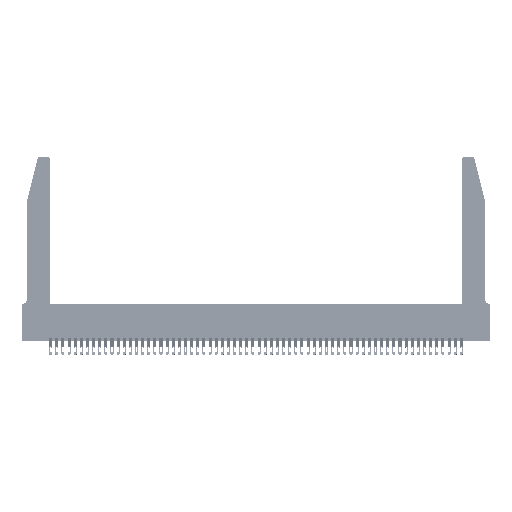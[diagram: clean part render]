
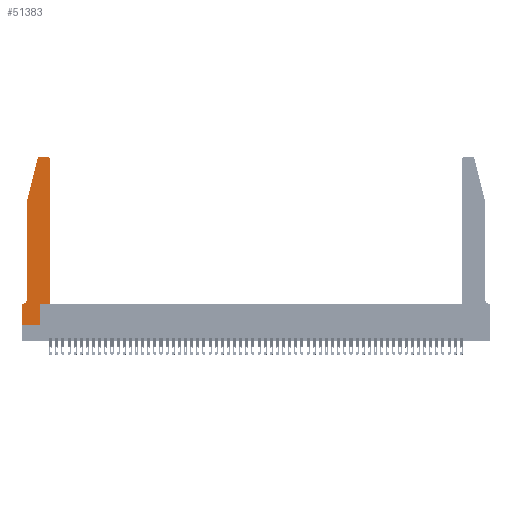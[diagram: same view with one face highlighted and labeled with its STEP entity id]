
A CAD part, top view. The second image highlights one B-rep face of the part: STEP entity #51383.
In plain terms, the highlighted planar face has unit normal (0, 0, 1).
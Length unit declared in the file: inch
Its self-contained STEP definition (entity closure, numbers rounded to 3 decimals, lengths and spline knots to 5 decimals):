
#634 = DIRECTION ( 'NONE',  ( 1., 0., 0. ) ) ;
#1074 = DIRECTION ( 'NONE',  ( -1., 0., 0. ) ) ;
#1122 = EDGE_CURVE ( 'NONE', #22611, #48524, #22011, .T. ) ;
#1380 = LINE ( 'NONE', #47984, #33876 ) ;
#1394 = DIRECTION ( 'NONE',  ( 1., 0., 0. ) ) ;
#1441 = DIRECTION ( 'NONE',  ( 1., 0., 0. ) ) ;
#1552 = EDGE_CURVE ( 'NONE', #48524, #32645, #35868, .T. ) ;
#1897 = DIRECTION ( 'NONE',  ( 1., 0., 0. ) ) ;
#2033 = LINE ( 'NONE', #38883, #20608 ) ;
#2248 = ORIENTED_EDGE ( 'NONE', *, *, #34589, .T. ) ;
#4146 = CARTESIAN_POINT ( 'NONE',  ( 0.4205, 2.75, 0.37 ) ) ;
#4470 = DIRECTION ( 'NONE',  ( 0., -1., 0. ) ) ;
#5925 = CARTESIAN_POINT ( 'NONE',  ( 0.4505, 0.35, 0.37 ) ) ;
#6037 = CARTESIAN_POINT ( 'NONE',  ( 0.0755, 2., 0.37 ) ) ;
#6945 = CARTESIAN_POINT ( 'NONE',  ( 0., 0., 0.37 ) ) ;
#9640 = VECTOR ( 'NONE', #28130, 39.37008 ) ;
#9688 = CARTESIAN_POINT ( 'NONE',  ( 0.4505, 2.72, 0.37 ) ) ;
#9996 = DIRECTION ( 'NONE',  ( 0., 0., 1. ) ) ;
#10215 = CARTESIAN_POINT ( 'NONE',  ( 0.2865, 0.35, 0.37 ) ) ;
#10845 = VERTEX_POINT ( 'NONE', #4146 ) ;
#10889 = LINE ( 'NONE', #16915, #42019 ) ;
#11600 = EDGE_CURVE ( 'NONE', #10845, #16654, #2033, .T. ) ;
#11763 = VECTOR ( 'NONE', #35792, 39.37008 ) ;
#12151 = CARTESIAN_POINT ( 'NONE',  ( 0., 0.35, 0.37 ) ) ;
#13722 = AXIS2_PLACEMENT_3D ( 'NONE', #47189, #35130, #1394 ) ;
#14450 = DIRECTION ( 'NONE',  ( 0., 1., 0. ) ) ;
#14862 = VECTOR ( 'NONE', #52957, 39.37008 ) ;
#14934 = LINE ( 'NONE', #52282, #9640 ) ;
#15047 = DIRECTION ( 'NONE',  ( 0., 0., 1. ) ) ;
#15683 = DIRECTION ( 'NONE',  ( 0., 0., -1. ) ) ;
#15743 = LINE ( 'NONE', #48577, #11763 ) ;
#16171 = CIRCLE ( 'NONE', #44896, 0.03 ) ;
#16654 = VERTEX_POINT ( 'NONE', #47803 ) ;
#16915 = CARTESIAN_POINT ( 'NONE',  ( 0.0755, 0.35, 0.37 ) ) ;
#19220 = FACE_OUTER_BOUND ( 'NONE', #26152, .T. ) ;
#20519 = VERTEX_POINT ( 'NONE', #49483 ) ;
#20608 = VECTOR ( 'NONE', #1074, 39.37008 ) ;
#20613 = CARTESIAN_POINT ( 'NONE',  ( 0.4505, 0.35, 0.37 ) ) ;
#21915 = LINE ( 'NONE', #5925, #41755 ) ;
#22011 = LINE ( 'NONE', #51734, #51879 ) ;
#22611 = VERTEX_POINT ( 'NONE', #27325 ) ;
#22914 = EDGE_CURVE ( 'NONE', #40343, #46086, #21915, .T. ) ;
#25844 = ORIENTED_EDGE ( 'NONE', *, *, #22914, .T. ) ;
#25861 = CARTESIAN_POINT ( 'NONE',  ( 0.4505, 0.35, 0.37 ) ) ;
#26067 = PLANE ( 'NONE',  #13722 ) ;
#26152 = EDGE_LOOP ( 'NONE', ( #49220, #48592, #42575, #53162, #42319, #46544, #34204, #2248, #26347, #48684, #25844, #44415 ) ) ;
#26347 = ORIENTED_EDGE ( 'NONE', *, *, #44273, .T. ) ;
#26510 = VERTEX_POINT ( 'NONE', #45526 ) ;
#26531 = VERTEX_POINT ( 'NONE', #12151 ) ;
#27325 = CARTESIAN_POINT ( 'NONE',  ( 0.0755, 2., 0.37 ) ) ;
#28130 = DIRECTION ( 'NONE',  ( 1., 0., 0. ) ) ;
#30059 = DIRECTION ( 'NONE',  ( -1., 0., 0. ) ) ;
#31421 = EDGE_CURVE ( 'NONE', #53577, #40343, #33157, .T. ) ;
#31683 = DIRECTION ( 'NONE',  ( 0., -1., 0. ) ) ;
#31684 = CIRCLE ( 'NONE', #46049, 0.03 ) ;
#32095 = LINE ( 'NONE', #6037, #14862 ) ;
#32645 = VERTEX_POINT ( 'NONE', #37017 ) ;
#33157 = LINE ( 'NONE', #25861, #43093 ) ;
#33876 = VECTOR ( 'NONE', #31683, 39.37008 ) ;
#34204 = ORIENTED_EDGE ( 'NONE', *, *, #50843, .T. ) ;
#34589 = EDGE_CURVE ( 'NONE', #48165, #20519, #14934, .T. ) ;
#34698 = CARTESIAN_POINT ( 'NONE',  ( 0.0755, 0.42, 0.37 ) ) ;
#35130 = DIRECTION ( 'NONE',  ( 0., 0., 1. ) ) ;
#35378 = EDGE_CURVE ( 'NONE', #26510, #22611, #32095, .T. ) ;
#35792 = DIRECTION ( 'NONE',  ( 0., 1., 0. ) ) ;
#35868 = CIRCLE ( 'NONE', #54213, 0.07 ) ;
#36995 = DIRECTION ( 'NONE',  ( -1., 0., 0. ) ) ;
#37017 = CARTESIAN_POINT ( 'NONE',  ( 0.0055, 0.35, 0.37 ) ) ;
#38326 = EDGE_CURVE ( 'NONE', #46086, #10845, #31684, .T. ) ;
#38883 = CARTESIAN_POINT ( 'NONE',  ( 0.2605, 2.75, 0.37 ) ) ;
#39867 = CARTESIAN_POINT ( 'NONE',  ( 0.4205, 2.72, 0.37 ) ) ;
#40343 = VERTEX_POINT ( 'NONE', #20613 ) ;
#40391 = EDGE_CURVE ( 'NONE', #32645, #26531, #10889, .T. ) ;
#41755 = VECTOR ( 'NONE', #14450, 39.37008 ) ;
#42019 = VECTOR ( 'NONE', #30059, 39.37008 ) ;
#42319 = ORIENTED_EDGE ( 'NONE', *, *, #1552, .T. ) ;
#42575 = ORIENTED_EDGE ( 'NONE', *, *, #35378, .T. ) ;
#43093 = VECTOR ( 'NONE', #634, 39.37008 ) ;
#43704 = CARTESIAN_POINT ( 'NONE',  ( 0.284, 2.72, 0.37 ) ) ;
#44273 = EDGE_CURVE ( 'NONE', #20519, #53577, #15743, .T. ) ;
#44415 = ORIENTED_EDGE ( 'NONE', *, *, #38326, .T. ) ;
#44896 = AXIS2_PLACEMENT_3D ( 'NONE', #43704, #9996, #1441 ) ;
#45173 = CARTESIAN_POINT ( 'NONE',  ( 0.0055, 0.42, 0.37 ) ) ;
#45526 = CARTESIAN_POINT ( 'NONE',  ( 0.25487, 2.72718, 0.37 ) ) ;
#46049 = AXIS2_PLACEMENT_3D ( 'NONE', #39867, #15047, #1897 ) ;
#46086 = VERTEX_POINT ( 'NONE', #9688 ) ;
#46544 = ORIENTED_EDGE ( 'NONE', *, *, #40391, .T. ) ;
#47189 = CARTESIAN_POINT ( 'NONE',  ( 0., 0.35, 0.37 ) ) ;
#47803 = CARTESIAN_POINT ( 'NONE',  ( 0.284, 2.75, 0.37 ) ) ;
#47984 = CARTESIAN_POINT ( 'NONE',  ( 0., 0., 0.37 ) ) ;
#48165 = VERTEX_POINT ( 'NONE', #6945 ) ;
#48524 = VERTEX_POINT ( 'NONE', #34698 ) ;
#48577 = CARTESIAN_POINT ( 'NONE',  ( 0.2865, 0.35, 0.37 ) ) ;
#48592 = ORIENTED_EDGE ( 'NONE', *, *, #49198, .T. ) ;
#48684 = ORIENTED_EDGE ( 'NONE', *, *, #31421, .T. ) ;
#49198 = EDGE_CURVE ( 'NONE', #16654, #26510, #16171, .T. ) ;
#49220 = ORIENTED_EDGE ( 'NONE', *, *, #11600, .T. ) ;
#49483 = CARTESIAN_POINT ( 'NONE',  ( 0.2865, 0., 0.37 ) ) ;
#50843 = EDGE_CURVE ( 'NONE', #26531, #48165, #1380, .T. ) ;
#51383 = ADVANCED_FACE ( 'NONE', ( #19220 ), #26067, .T. ) ;
#51734 = CARTESIAN_POINT ( 'NONE',  ( 0.0755, 2., 0.37 ) ) ;
#51879 = VECTOR ( 'NONE', #4470, 39.37008 ) ;
#52282 = CARTESIAN_POINT ( 'NONE',  ( 0., 0., 0.37 ) ) ;
#52957 = DIRECTION ( 'NONE',  ( -0.239, -0.971, 0. ) ) ;
#53162 = ORIENTED_EDGE ( 'NONE', *, *, #1122, .T. ) ;
#53577 = VERTEX_POINT ( 'NONE', #10215 ) ;
#54213 = AXIS2_PLACEMENT_3D ( 'NONE', #45173, #15683, #36995 ) ;
